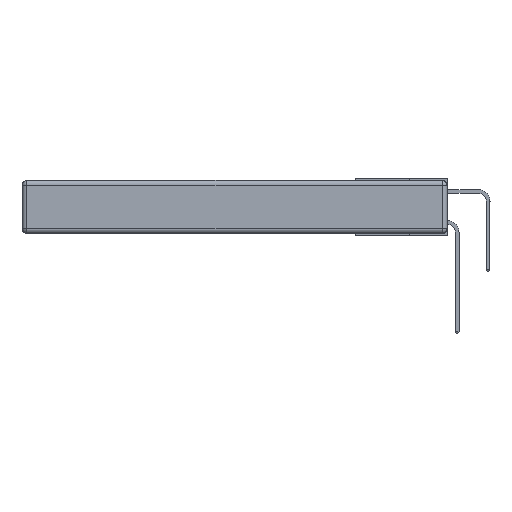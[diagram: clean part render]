
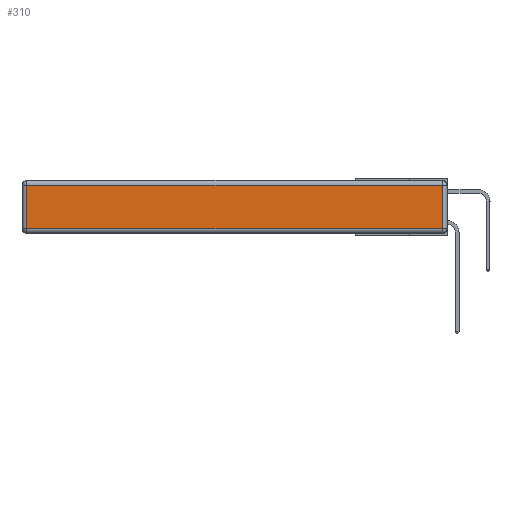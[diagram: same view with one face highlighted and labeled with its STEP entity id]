
A CAD part, left-side view. The second image highlights one B-rep face of the part: STEP entity #310.
In plain terms, the highlighted planar face has unit normal (-1, 0, 0).
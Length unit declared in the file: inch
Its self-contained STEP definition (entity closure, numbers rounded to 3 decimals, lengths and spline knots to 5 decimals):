
#310 = ADVANCED_FACE ( 'NONE', ( #4694 ), #4389, .T. ) ;
#471 = DIRECTION ( 'NONE',  ( 0., -1., 0. ) ) ;
#668 = VERTEX_POINT ( 'NONE', #8664 ) ;
#2180 = VECTOR ( 'NONE', #17473, 39.37008 ) ;
#3589 = LINE ( 'NONE', #10409, #21349 ) ;
#4315 = DIRECTION ( 'NONE',  ( 0., 0., 1. ) ) ;
#4389 = PLANE ( 'NONE',  #10356 ) ;
#4571 = ORIENTED_EDGE ( 'NONE', *, *, #22064, .T. ) ;
#4694 = FACE_OUTER_BOUND ( 'NONE', #6711, .T. ) ;
#5453 = CARTESIAN_POINT ( 'NONE',  ( 0., 2.75, -0.03 ) ) ;
#5900 = VERTEX_POINT ( 'NONE', #13237 ) ;
#6277 = DIRECTION ( 'NONE',  ( -1., 0., 0. ) ) ;
#6711 = EDGE_LOOP ( 'NONE', ( #19312, #6942, #4571, #15349 ) ) ;
#6793 = LINE ( 'NONE', #5453, #2180 ) ;
#6942 = ORIENTED_EDGE ( 'NONE', *, *, #21395, .T. ) ;
#7468 = VECTOR ( 'NONE', #12139, 39.37008 ) ;
#7675 = CARTESIAN_POINT ( 'NONE',  ( 0., 0.03, -0.03 ) ) ;
#8664 = CARTESIAN_POINT ( 'NONE',  ( 0., 2.72, -0.03 ) ) ;
#8752 = DIRECTION ( 'NONE',  ( 0., 0., 1. ) ) ;
#10356 = AXIS2_PLACEMENT_3D ( 'NONE', #18142, #6277, #4315 ) ;
#10409 = CARTESIAN_POINT ( 'NONE',  ( 0., 0.03, -0.343 ) ) ;
#12139 = DIRECTION ( 'NONE',  ( 0., 0., -1. ) ) ;
#13237 = CARTESIAN_POINT ( 'NONE',  ( 0., 2.72, -0.313 ) ) ;
#14901 = EDGE_CURVE ( 'NONE', #5900, #19266, #22156, .T. ) ;
#15349 = ORIENTED_EDGE ( 'NONE', *, *, #18938, .T. ) ;
#15725 = VERTEX_POINT ( 'NONE', #7675 ) ;
#17022 = VECTOR ( 'NONE', #471, 39.37008 ) ;
#17171 = CARTESIAN_POINT ( 'NONE',  ( 0., 2.72, -0.343 ) ) ;
#17473 = DIRECTION ( 'NONE',  ( 0., 1., 0. ) ) ;
#17949 = LINE ( 'NONE', #17171, #7468 ) ;
#18142 = CARTESIAN_POINT ( 'NONE',  ( 0., 0., -0.343 ) ) ;
#18938 = EDGE_CURVE ( 'NONE', #668, #5900, #17949, .T. ) ;
#19266 = VERTEX_POINT ( 'NONE', #19361 ) ;
#19312 = ORIENTED_EDGE ( 'NONE', *, *, #14901, .T. ) ;
#19361 = CARTESIAN_POINT ( 'NONE',  ( 0., 0.03, -0.313 ) ) ;
#21054 = CARTESIAN_POINT ( 'NONE',  ( 0., 0., -0.313 ) ) ;
#21349 = VECTOR ( 'NONE', #8752, 39.37008 ) ;
#21395 = EDGE_CURVE ( 'NONE', #19266, #15725, #3589, .T. ) ;
#22064 = EDGE_CURVE ( 'NONE', #15725, #668, #6793, .T. ) ;
#22156 = LINE ( 'NONE', #21054, #17022 ) ;
